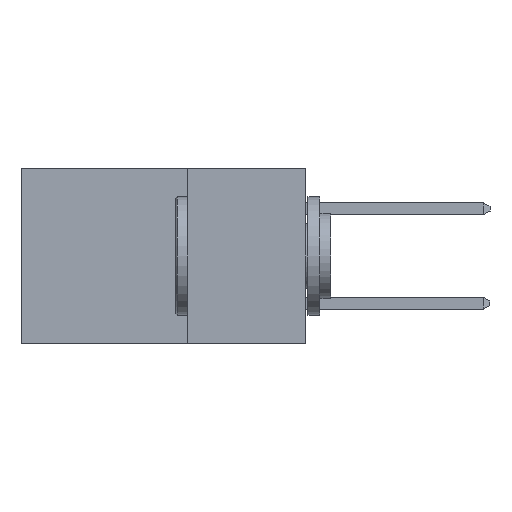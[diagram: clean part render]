
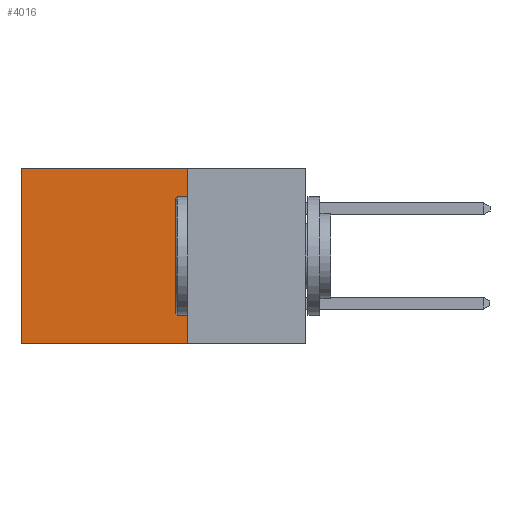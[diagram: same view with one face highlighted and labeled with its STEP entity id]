
A CAD part, left-side view. The second image highlights one B-rep face of the part: STEP entity #4016.
In plain terms, the highlighted planar face has unit normal (-1, 0, 0).
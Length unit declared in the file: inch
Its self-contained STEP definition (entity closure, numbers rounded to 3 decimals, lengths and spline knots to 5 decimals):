
#3303 = ORIENTED_EDGE ( 'NONE', *, *, #19757, .F. ) ;
#3321 = LINE ( 'NONE', #4237, #8132 ) ;
#3618 = ORIENTED_EDGE ( 'NONE', *, *, #16510, .T. ) ;
#4016 = ADVANCED_FACE ( 'NONE', ( #6581 ), #5023, .F. ) ;
#4184 = CARTESIAN_POINT ( 'NONE',  ( 0.298, 0.6, -0.37 ) ) ;
#4237 = CARTESIAN_POINT ( 'NONE',  ( 0.298, 0.6, 0. ) ) ;
#4449 = CARTESIAN_POINT ( 'NONE',  ( 0.298, 0.25, 0. ) ) ;
#4938 = ORIENTED_EDGE ( 'NONE', *, *, #18381, .F. ) ;
#5023 = PLANE ( 'NONE',  #21479 ) ;
#6177 = CARTESIAN_POINT ( 'NONE',  ( 0.298, 0.6, 0. ) ) ;
#6581 = FACE_OUTER_BOUND ( 'NONE', #22373, .T. ) ;
#6672 = CARTESIAN_POINT ( 'NONE',  ( 0.298, 0.25, 0. ) ) ;
#7390 = DIRECTION ( 'NONE',  ( 0., 1., 0. ) ) ;
#7610 = LINE ( 'NONE', #20166, #16218 ) ;
#8070 = LINE ( 'NONE', #8669, #22025 ) ;
#8132 = VECTOR ( 'NONE', #9736, 39.37008 ) ;
#8669 = CARTESIAN_POINT ( 'NONE',  ( 0.298, 0.25, 0. ) ) ;
#9736 = DIRECTION ( 'NONE',  ( 0., 0., -1. ) ) ;
#10528 = DIRECTION ( 'NONE',  ( 1., 0., 0. ) ) ;
#11380 = EDGE_CURVE ( 'NONE', #21219, #19731, #8070, .T. ) ;
#12934 = CARTESIAN_POINT ( 'NONE',  ( 0.298, 0.25, -0.37 ) ) ;
#13836 = LINE ( 'NONE', #4449, #18695 ) ;
#15377 = VERTEX_POINT ( 'NONE', #12934 ) ;
#15421 = ORIENTED_EDGE ( 'NONE', *, *, #11380, .T. ) ;
#15943 = CARTESIAN_POINT ( 'NONE',  ( 0.298, 0.25, 0. ) ) ;
#16218 = VECTOR ( 'NONE', #7390, 39.37008 ) ;
#16510 = EDGE_CURVE ( 'NONE', #19731, #17832, #3321, .T. ) ;
#17832 = VERTEX_POINT ( 'NONE', #4184 ) ;
#17860 = DIRECTION ( 'NONE',  ( 0., 1., 0. ) ) ;
#18381 = EDGE_CURVE ( 'NONE', #15377, #17832, #7610, .T. ) ;
#18695 = VECTOR ( 'NONE', #18942, 39.37008 ) ;
#18942 = DIRECTION ( 'NONE',  ( 0., 0., -1. ) ) ;
#19731 = VERTEX_POINT ( 'NONE', #6177 ) ;
#19757 = EDGE_CURVE ( 'NONE', #21219, #15377, #13836, .T. ) ;
#20166 = CARTESIAN_POINT ( 'NONE',  ( 0.298, 0.25, -0.37 ) ) ;
#21219 = VERTEX_POINT ( 'NONE', #6672 ) ;
#21479 = AXIS2_PLACEMENT_3D ( 'NONE', #15943, #10528, #23177 ) ;
#22025 = VECTOR ( 'NONE', #17860, 39.37008 ) ;
#22373 = EDGE_LOOP ( 'NONE', ( #3618, #4938, #3303, #15421 ) ) ;
#23177 = DIRECTION ( 'NONE',  ( 0., 0., -1. ) ) ;
